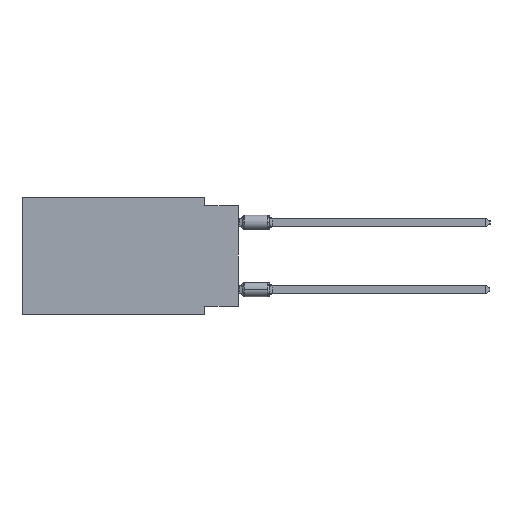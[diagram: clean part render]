
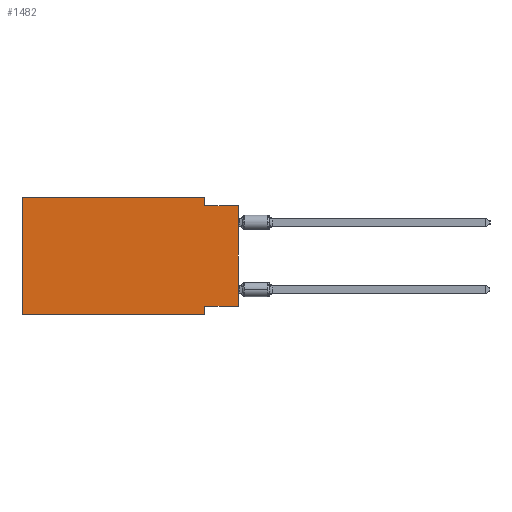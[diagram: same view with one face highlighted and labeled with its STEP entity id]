
A CAD part, left-side view. The second image highlights one B-rep face of the part: STEP entity #1482.
In plain terms, the highlighted planar face has unit normal (-1, 0, 0).
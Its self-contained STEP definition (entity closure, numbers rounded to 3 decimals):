
#176 = VERTEX_POINT ( 'NONE', #13138 ) ;
#328 = LINE ( 'NONE', #10681, #1311 ) ;
#420 = ORIENTED_EDGE ( 'NONE', *, *, #15200, .F. ) ;
#518 = VECTOR ( 'NONE', #18475, 1000. ) ;
#732 = CARTESIAN_POINT ( 'NONE',  ( 0., 2.54, 0. ) ) ;
#1165 = CARTESIAN_POINT ( 'NONE',  ( 0., 16.383, -8.89 ) ) ;
#1224 = EDGE_CURVE ( 'NONE', #5337, #4227, #7596, .T. ) ;
#1311 = VECTOR ( 'NONE', #6019, 1000. ) ;
#1438 = EDGE_LOOP ( 'NONE', ( #10828, #420, #15301, #17489, #12150, #4357, #10611, #17033 ) ) ;
#1482 = ADVANCED_FACE ( 'NONE', ( #17930 ), #17830, .F. ) ;
#2032 = CARTESIAN_POINT ( 'NONE',  ( 0., 2.54, -0.635 ) ) ;
#2579 = CARTESIAN_POINT ( 'NONE',  ( 0., 2.54, 0. ) ) ;
#2684 = DIRECTION ( 'NONE',  ( 0., 0., -1. ) ) ;
#2757 = EDGE_CURVE ( 'NONE', #176, #16575, #328, .T. ) ;
#2810 = AXIS2_PLACEMENT_3D ( 'NONE', #8960, #4184, #2684 ) ;
#2834 = VECTOR ( 'NONE', #3872, 1000. ) ;
#3850 = DIRECTION ( 'NONE',  ( 0., 0., 1. ) ) ;
#3872 = DIRECTION ( 'NONE',  ( 0., -1., 0. ) ) ;
#4055 = DIRECTION ( 'NONE',  ( 0., 1., 0. ) ) ;
#4184 = DIRECTION ( 'NONE',  ( 1., 0., 0. ) ) ;
#4227 = VERTEX_POINT ( 'NONE', #732 ) ;
#4357 = ORIENTED_EDGE ( 'NONE', *, *, #16916, .T. ) ;
#5337 = VERTEX_POINT ( 'NONE', #9791 ) ;
#5339 = CARTESIAN_POINT ( 'NONE',  ( 0., 0., 0. ) ) ;
#5465 = CARTESIAN_POINT ( 'NONE',  ( 0., 0., -8.255 ) ) ;
#5627 = VERTEX_POINT ( 'NONE', #12843 ) ;
#5948 = EDGE_CURVE ( 'NONE', #16428, #5627, #6838, .T. ) ;
#6019 = DIRECTION ( 'NONE',  ( 0., 0., -1. ) ) ;
#6637 = VECTOR ( 'NONE', #4055, 1000. ) ;
#6838 = LINE ( 'NONE', #5339, #7160 ) ;
#7160 = VECTOR ( 'NONE', #3850, 1000. ) ;
#7205 = VERTEX_POINT ( 'NONE', #1165 ) ;
#7358 = LINE ( 'NONE', #5465, #6637 ) ;
#7441 = VERTEX_POINT ( 'NONE', #2032 ) ;
#7596 = LINE ( 'NONE', #12187, #14608 ) ;
#8960 = CARTESIAN_POINT ( 'NONE',  ( 0., 16.383, 0. ) ) ;
#9791 = CARTESIAN_POINT ( 'NONE',  ( 0., 16.383, 0. ) ) ;
#10611 = ORIENTED_EDGE ( 'NONE', *, *, #2757, .F. ) ;
#10681 = CARTESIAN_POINT ( 'NONE',  ( 0., 2.54, -8.89 ) ) ;
#10760 = LINE ( 'NONE', #10959, #12275 ) ;
#10828 = ORIENTED_EDGE ( 'NONE', *, *, #5948, .T. ) ;
#10959 = CARTESIAN_POINT ( 'NONE',  ( 0., 0., -0.635 ) ) ;
#11339 = LINE ( 'NONE', #18895, #2834 ) ;
#12150 = ORIENTED_EDGE ( 'NONE', *, *, #15667, .F. ) ;
#12187 = CARTESIAN_POINT ( 'NONE',  ( 0., 16.383, 0. ) ) ;
#12275 = VECTOR ( 'NONE', #14052, 1000. ) ;
#12406 = CARTESIAN_POINT ( 'NONE',  ( 0., 16.383, 0. ) ) ;
#12843 = CARTESIAN_POINT ( 'NONE',  ( 0., 0., -0.635 ) ) ;
#13138 = CARTESIAN_POINT ( 'NONE',  ( 0., 2.54, -8.255 ) ) ;
#14052 = DIRECTION ( 'NONE',  ( 0., -1., 0. ) ) ;
#14071 = EDGE_CURVE ( 'NONE', #4227, #7441, #17516, .T. ) ;
#14549 = CARTESIAN_POINT ( 'NONE',  ( 0., 2.54, -8.89 ) ) ;
#14608 = VECTOR ( 'NONE', #18336, 1000. ) ;
#15200 = EDGE_CURVE ( 'NONE', #7441, #5627, #10760, .T. ) ;
#15301 = ORIENTED_EDGE ( 'NONE', *, *, #14071, .F. ) ;
#15667 = EDGE_CURVE ( 'NONE', #7205, #5337, #18564, .T. ) ;
#16428 = VERTEX_POINT ( 'NONE', #18429 ) ;
#16575 = VERTEX_POINT ( 'NONE', #14549 ) ;
#16916 = EDGE_CURVE ( 'NONE', #7205, #16575, #11339, .T. ) ;
#17033 = ORIENTED_EDGE ( 'NONE', *, *, #18864, .F. ) ;
#17384 = VECTOR ( 'NONE', #17615, 1000. ) ;
#17489 = ORIENTED_EDGE ( 'NONE', *, *, #1224, .F. ) ;
#17516 = LINE ( 'NONE', #2579, #17384 ) ;
#17615 = DIRECTION ( 'NONE',  ( 0., 0., -1. ) ) ;
#17830 = PLANE ( 'NONE',  #2810 ) ;
#17930 = FACE_OUTER_BOUND ( 'NONE', #1438, .T. ) ;
#18336 = DIRECTION ( 'NONE',  ( 0., -1., 0. ) ) ;
#18429 = CARTESIAN_POINT ( 'NONE',  ( 0., 0., -8.255 ) ) ;
#18475 = DIRECTION ( 'NONE',  ( 0., 0., 1. ) ) ;
#18564 = LINE ( 'NONE', #12406, #518 ) ;
#18864 = EDGE_CURVE ( 'NONE', #16428, #176, #7358, .T. ) ;
#18895 = CARTESIAN_POINT ( 'NONE',  ( 0., 16.383, -8.89 ) ) ;
